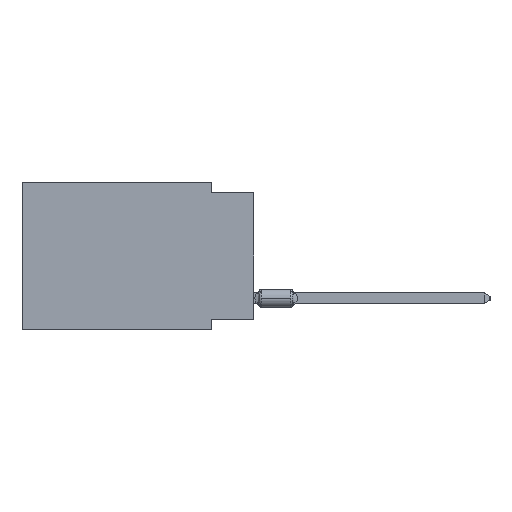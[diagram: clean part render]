
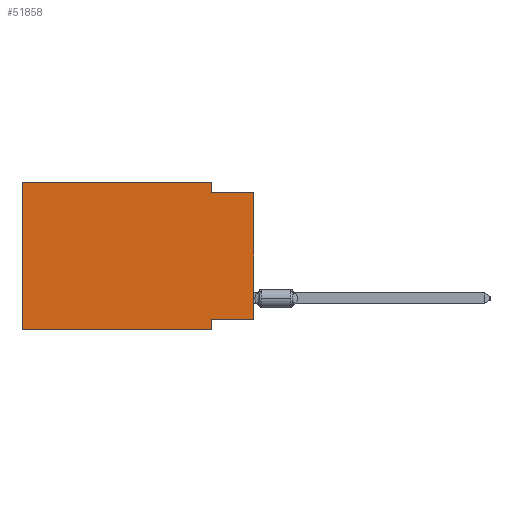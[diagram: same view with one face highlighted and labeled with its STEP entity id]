
A CAD part, left-side view. The second image highlights one B-rep face of the part: STEP entity #51858.
In plain terms, the highlighted planar face has unit normal (-1, 0, 0).
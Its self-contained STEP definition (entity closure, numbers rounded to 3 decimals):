
#1862 = CARTESIAN_POINT ( 'NONE',  ( 0., 13.97, 0. ) ) ;
#2096 = VECTOR ( 'NONE', #8071, 1000. ) ;
#2538 = ORIENTED_EDGE ( 'NONE', *, *, #32970, .F. ) ;
#3413 = ORIENTED_EDGE ( 'NONE', *, *, #31927, .F. ) ;
#3554 = CARTESIAN_POINT ( 'NONE',  ( 0., 0., -0.635 ) ) ;
#5826 = VERTEX_POINT ( 'NONE', #52108 ) ;
#6255 = VERTEX_POINT ( 'NONE', #19305 ) ;
#6695 = DIRECTION ( 'NONE',  ( 0., 0., 1. ) ) ;
#6877 = DIRECTION ( 'NONE',  ( 0., 0., -1. ) ) ;
#7121 = VECTOR ( 'NONE', #6877, 1000. ) ;
#8071 = DIRECTION ( 'NONE',  ( 0., 1., 0. ) ) ;
#8487 = VECTOR ( 'NONE', #30514, 1000. ) ;
#10287 = VERTEX_POINT ( 'NONE', #3554 ) ;
#10927 = LINE ( 'NONE', #51010, #42342 ) ;
#11066 = FACE_OUTER_BOUND ( 'NONE', #52877, .T. ) ;
#11138 = EDGE_CURVE ( 'NONE', #43073, #6255, #48538, .T. ) ;
#11393 = LINE ( 'NONE', #32861, #31830 ) ;
#12558 = VECTOR ( 'NONE', #35950, 1000. ) ;
#13437 = CARTESIAN_POINT ( 'NONE',  ( 0., 2.54, -8.255 ) ) ;
#14197 = EDGE_CURVE ( 'NONE', #21075, #10287, #28708, .T. ) ;
#15339 = VERTEX_POINT ( 'NONE', #34640 ) ;
#16077 = CARTESIAN_POINT ( 'NONE',  ( 0., 2.54, 0. ) ) ;
#19305 = CARTESIAN_POINT ( 'NONE',  ( 0., 2.54, -8.89 ) ) ;
#20087 = CARTESIAN_POINT ( 'NONE',  ( 0., 0., 0. ) ) ;
#21075 = VERTEX_POINT ( 'NONE', #50472 ) ;
#22582 = EDGE_CURVE ( 'NONE', #21075, #28861, #41310, .T. ) ;
#25611 = DIRECTION ( 'NONE',  ( 0., -1., 0. ) ) ;
#27265 = DIRECTION ( 'NONE',  ( 0., 0., -1. ) ) ;
#28072 = PLANE ( 'NONE',  #28928 ) ;
#28112 = CARTESIAN_POINT ( 'NONE',  ( 0., 13.97, -8.89 ) ) ;
#28708 = LINE ( 'NONE', #20087, #30656 ) ;
#28861 = VERTEX_POINT ( 'NONE', #13437 ) ;
#28927 = DIRECTION ( 'NONE',  ( 0., 0., 1. ) ) ;
#28928 = AXIS2_PLACEMENT_3D ( 'NONE', #1862, #44299, #53763 ) ;
#29623 = ORIENTED_EDGE ( 'NONE', *, *, #22582, .F. ) ;
#29898 = ORIENTED_EDGE ( 'NONE', *, *, #31245, .F. ) ;
#30514 = DIRECTION ( 'NONE',  ( 0., -1., 0. ) ) ;
#30656 = VECTOR ( 'NONE', #6695, 1000. ) ;
#31245 = EDGE_CURVE ( 'NONE', #15339, #5826, #47020, .T. ) ;
#31382 = VERTEX_POINT ( 'NONE', #31625 ) ;
#31625 = CARTESIAN_POINT ( 'NONE',  ( 0., 2.54, -0.635 ) ) ;
#31830 = VECTOR ( 'NONE', #28927, 1000. ) ;
#31927 = EDGE_CURVE ( 'NONE', #43073, #15339, #11393, .T. ) ;
#32396 = VECTOR ( 'NONE', #27265, 1000. ) ;
#32861 = CARTESIAN_POINT ( 'NONE',  ( 0., 13.97, 0. ) ) ;
#32970 = EDGE_CURVE ( 'NONE', #28861, #6255, #48512, .T. ) ;
#33709 = ORIENTED_EDGE ( 'NONE', *, *, #40519, .F. ) ;
#34640 = CARTESIAN_POINT ( 'NONE',  ( 0., 13.97, 0. ) ) ;
#34725 = CARTESIAN_POINT ( 'NONE',  ( 0., 13.97, 0. ) ) ;
#35950 = DIRECTION ( 'NONE',  ( 0., -1., 0. ) ) ;
#37318 = ORIENTED_EDGE ( 'NONE', *, *, #11138, .T. ) ;
#40519 = EDGE_CURVE ( 'NONE', #5826, #31382, #53226, .T. ) ;
#41310 = LINE ( 'NONE', #50227, #2096 ) ;
#41493 = CARTESIAN_POINT ( 'NONE',  ( 0., 13.97, -8.89 ) ) ;
#42342 = VECTOR ( 'NONE', #25611, 1000. ) ;
#43073 = VERTEX_POINT ( 'NONE', #41493 ) ;
#44299 = DIRECTION ( 'NONE',  ( 1., 0., 0. ) ) ;
#47020 = LINE ( 'NONE', #34725, #8487 ) ;
#47722 = ORIENTED_EDGE ( 'NONE', *, *, #14197, .T. ) ;
#48512 = LINE ( 'NONE', #49338, #32396 ) ;
#48538 = LINE ( 'NONE', #28112, #12558 ) ;
#49152 = ORIENTED_EDGE ( 'NONE', *, *, #51606, .F. ) ;
#49338 = CARTESIAN_POINT ( 'NONE',  ( 0., 2.54, -8.89 ) ) ;
#50227 = CARTESIAN_POINT ( 'NONE',  ( 0., 0., -8.255 ) ) ;
#50472 = CARTESIAN_POINT ( 'NONE',  ( 0., 0., -8.255 ) ) ;
#51010 = CARTESIAN_POINT ( 'NONE',  ( 0., 0., -0.635 ) ) ;
#51606 = EDGE_CURVE ( 'NONE', #31382, #10287, #10927, .T. ) ;
#51858 = ADVANCED_FACE ( 'NONE', ( #11066 ), #28072, .F. ) ;
#52108 = CARTESIAN_POINT ( 'NONE',  ( 0., 2.54, 0. ) ) ;
#52877 = EDGE_LOOP ( 'NONE', ( #47722, #49152, #33709, #29898, #3413, #37318, #2538, #29623 ) ) ;
#53226 = LINE ( 'NONE', #16077, #7121 ) ;
#53763 = DIRECTION ( 'NONE',  ( 0., 0., -1. ) ) ;
